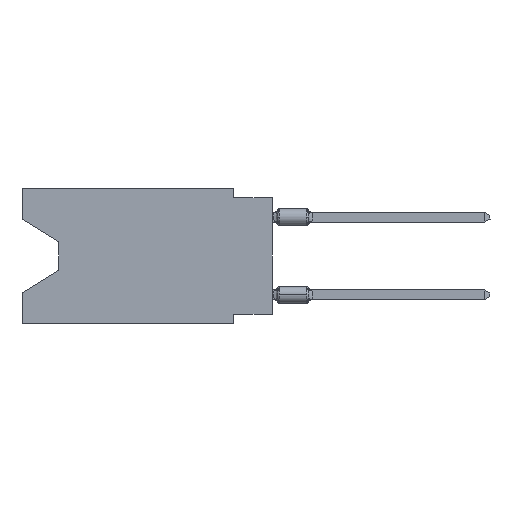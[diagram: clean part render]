
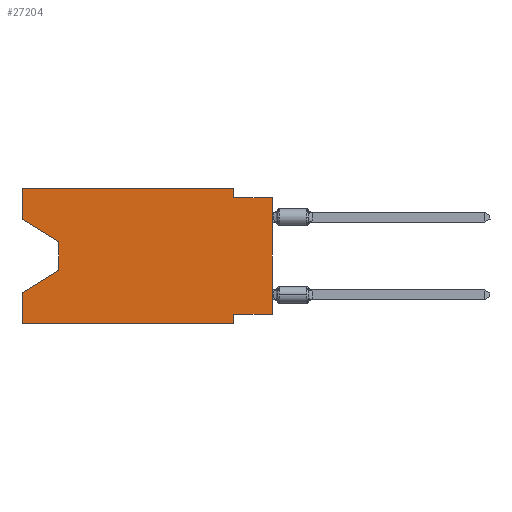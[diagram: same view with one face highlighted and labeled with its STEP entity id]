
A CAD part, left-side view. The second image highlights one B-rep face of the part: STEP entity #27204.
In plain terms, the highlighted planar face has unit normal (-1, 0, 0).
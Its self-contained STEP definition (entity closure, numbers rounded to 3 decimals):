
#1411 = LINE ( 'NONE', #23694, #12501 ) ;
#1757 = CARTESIAN_POINT ( 'NONE',  ( 0., 16.383, -2.038 ) ) ;
#1814 = CARTESIAN_POINT ( 'NONE',  ( 0., 2.54, -8.89 ) ) ;
#2016 = ORIENTED_EDGE ( 'NONE', *, *, #4194, .F. ) ;
#2137 = CARTESIAN_POINT ( 'NONE',  ( 0., 13.97, -3.505 ) ) ;
#2566 = ORIENTED_EDGE ( 'NONE', *, *, #7292, .F. ) ;
#2676 = ORIENTED_EDGE ( 'NONE', *, *, #3734, .F. ) ;
#3018 = ORIENTED_EDGE ( 'NONE', *, *, #24807, .T. ) ;
#3064 = VERTEX_POINT ( 'NONE', #33294 ) ;
#3185 = CARTESIAN_POINT ( 'NONE',  ( 0., 13.97, -5.385 ) ) ;
#3734 = EDGE_CURVE ( 'NONE', #14768, #6152, #21163, .T. ) ;
#4187 = LINE ( 'NONE', #35355, #20433 ) ;
#4194 = EDGE_CURVE ( 'NONE', #21280, #28061, #1411, .T. ) ;
#4220 = CARTESIAN_POINT ( 'NONE',  ( 0., 0., -0.635 ) ) ;
#4447 = ORIENTED_EDGE ( 'NONE', *, *, #34092, .T. ) ;
#4847 = VECTOR ( 'NONE', #28976, 1000. ) ;
#4912 = VERTEX_POINT ( 'NONE', #12279 ) ;
#5287 = ORIENTED_EDGE ( 'NONE', *, *, #12831, .F. ) ;
#5660 = DIRECTION ( 'NONE',  ( 0., 0., -1. ) ) ;
#6021 = CARTESIAN_POINT ( 'NONE',  ( 0., 0., -8.255 ) ) ;
#6152 = VERTEX_POINT ( 'NONE', #8981 ) ;
#6333 = VECTOR ( 'NONE', #27200, 1000. ) ;
#7092 = CARTESIAN_POINT ( 'NONE',  ( 0., 16.383, -8.89 ) ) ;
#7292 = EDGE_CURVE ( 'NONE', #6152, #21280, #4187, .T. ) ;
#7341 = EDGE_CURVE ( 'NONE', #36723, #3064, #16434, .T. ) ;
#7371 = EDGE_CURVE ( 'NONE', #33607, #33467, #10858, .T. ) ;
#8981 = CARTESIAN_POINT ( 'NONE',  ( 0., 2.54, 0. ) ) ;
#9876 = FACE_OUTER_BOUND ( 'NONE', #21098, .T. ) ;
#10739 = EDGE_CURVE ( 'NONE', #34623, #33607, #20695, .T. ) ;
#10837 = DIRECTION ( 'NONE',  ( 0., 0.855, -0.519 ) ) ;
#10858 = LINE ( 'NONE', #2137, #31071 ) ;
#10965 = VERTEX_POINT ( 'NONE', #6021 ) ;
#11727 = VECTOR ( 'NONE', #29346, 1000. ) ;
#12279 = CARTESIAN_POINT ( 'NONE',  ( 0., 2.54, -8.255 ) ) ;
#12501 = VECTOR ( 'NONE', #32016, 1000. ) ;
#12659 = CARTESIAN_POINT ( 'NONE',  ( 0., 16.383, 0. ) ) ;
#12730 = DIRECTION ( 'NONE',  ( 0., -0.855, -0.519 ) ) ;
#12831 = EDGE_CURVE ( 'NONE', #10965, #4912, #28513, .T. ) ;
#12894 = CARTESIAN_POINT ( 'NONE',  ( 0., 16.383, 0. ) ) ;
#12972 = LINE ( 'NONE', #24276, #25467 ) ;
#13986 = AXIS2_PLACEMENT_3D ( 'NONE', #21547, #35648, #20819 ) ;
#14203 = ORIENTED_EDGE ( 'NONE', *, *, #35403, .F. ) ;
#14305 = ORIENTED_EDGE ( 'NONE', *, *, #10739, .T. ) ;
#14768 = VERTEX_POINT ( 'NONE', #12894 ) ;
#15359 = LINE ( 'NONE', #23704, #6333 ) ;
#16434 = LINE ( 'NONE', #22527, #22220 ) ;
#17777 = LINE ( 'NONE', #33458, #33851 ) ;
#18309 = CARTESIAN_POINT ( 'NONE',  ( 0., 16.383, -2.038 ) ) ;
#18396 = LINE ( 'NONE', #7092, #11727 ) ;
#19078 = DIRECTION ( 'NONE',  ( 0., 0., 1. ) ) ;
#20433 = VECTOR ( 'NONE', #33291, 1000. ) ;
#20695 = LINE ( 'NONE', #1757, #34856 ) ;
#20819 = DIRECTION ( 'NONE',  ( 0., 0., -1. ) ) ;
#21098 = EDGE_LOOP ( 'NONE', ( #14305, #26415, #31894, #22830, #3018, #31359, #5287, #4447, #2016, #2566, #2676, #14203 ) ) ;
#21160 = CARTESIAN_POINT ( 'NONE',  ( 0., 13.97, -3.505 ) ) ;
#21163 = LINE ( 'NONE', #12659, #4847 ) ;
#21280 = VERTEX_POINT ( 'NONE', #28754 ) ;
#21547 = CARTESIAN_POINT ( 'NONE',  ( 0., 16.383, 0. ) ) ;
#21590 = VERTEX_POINT ( 'NONE', #1814 ) ;
#22154 = VECTOR ( 'NONE', #33536, 1000. ) ;
#22220 = VECTOR ( 'NONE', #27371, 1000. ) ;
#22527 = CARTESIAN_POINT ( 'NONE',  ( 0., 16.383, 0. ) ) ;
#22618 = VECTOR ( 'NONE', #19078, 1000. ) ;
#22830 = ORIENTED_EDGE ( 'NONE', *, *, #7341, .F. ) ;
#23260 = EDGE_CURVE ( 'NONE', #4912, #21590, #15359, .T. ) ;
#23694 = CARTESIAN_POINT ( 'NONE',  ( 0., 0., -0.635 ) ) ;
#23704 = CARTESIAN_POINT ( 'NONE',  ( 0., 2.54, -8.89 ) ) ;
#24276 = CARTESIAN_POINT ( 'NONE',  ( 0., 16.383, 0. ) ) ;
#24653 = DIRECTION ( 'NONE',  ( 0., 0., 1. ) ) ;
#24807 = EDGE_CURVE ( 'NONE', #36723, #21590, #18396, .T. ) ;
#25467 = VECTOR ( 'NONE', #24653, 1000. ) ;
#26415 = ORIENTED_EDGE ( 'NONE', *, *, #7371, .T. ) ;
#26877 = CARTESIAN_POINT ( 'NONE',  ( 0., 0., 0. ) ) ;
#26906 = EDGE_CURVE ( 'NONE', #33467, #3064, #17777, .T. ) ;
#27124 = PLANE ( 'NONE',  #13986 ) ;
#27200 = DIRECTION ( 'NONE',  ( 0., 0., -1. ) ) ;
#27204 = ADVANCED_FACE ( 'NONE', ( #9876 ), #27124, .F. ) ;
#27371 = DIRECTION ( 'NONE',  ( 0., 0., 1. ) ) ;
#27603 = LINE ( 'NONE', #26877, #22618 ) ;
#27963 = CARTESIAN_POINT ( 'NONE',  ( 0., 0., -8.255 ) ) ;
#28061 = VERTEX_POINT ( 'NONE', #4220 ) ;
#28513 = LINE ( 'NONE', #27963, #22154 ) ;
#28754 = CARTESIAN_POINT ( 'NONE',  ( 0., 2.54, -0.635 ) ) ;
#28976 = DIRECTION ( 'NONE',  ( 0., -1., 0. ) ) ;
#29346 = DIRECTION ( 'NONE',  ( 0., -1., 0. ) ) ;
#31071 = VECTOR ( 'NONE', #5660, 1000. ) ;
#31359 = ORIENTED_EDGE ( 'NONE', *, *, #23260, .F. ) ;
#31894 = ORIENTED_EDGE ( 'NONE', *, *, #26906, .T. ) ;
#32016 = DIRECTION ( 'NONE',  ( 0., -1., 0. ) ) ;
#33291 = DIRECTION ( 'NONE',  ( 0., 0., -1. ) ) ;
#33294 = CARTESIAN_POINT ( 'NONE',  ( 0., 16.383, -6.852 ) ) ;
#33458 = CARTESIAN_POINT ( 'NONE',  ( 0., 13.97, -5.385 ) ) ;
#33467 = VERTEX_POINT ( 'NONE', #3185 ) ;
#33536 = DIRECTION ( 'NONE',  ( 0., 1., 0. ) ) ;
#33607 = VERTEX_POINT ( 'NONE', #21160 ) ;
#33851 = VECTOR ( 'NONE', #10837, 1000. ) ;
#34092 = EDGE_CURVE ( 'NONE', #10965, #28061, #27603, .T. ) ;
#34103 = CARTESIAN_POINT ( 'NONE',  ( 0., 16.383, -8.89 ) ) ;
#34623 = VERTEX_POINT ( 'NONE', #18309 ) ;
#34856 = VECTOR ( 'NONE', #12730, 1000. ) ;
#35355 = CARTESIAN_POINT ( 'NONE',  ( 0., 2.54, 0. ) ) ;
#35403 = EDGE_CURVE ( 'NONE', #34623, #14768, #12972, .T. ) ;
#35648 = DIRECTION ( 'NONE',  ( 1., 0., 0. ) ) ;
#36723 = VERTEX_POINT ( 'NONE', #34103 ) ;
